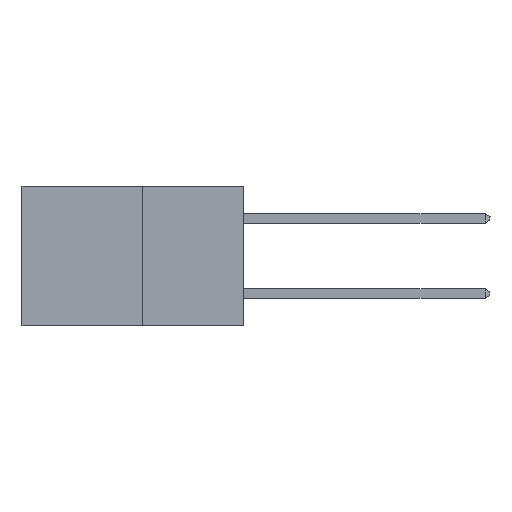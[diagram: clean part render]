
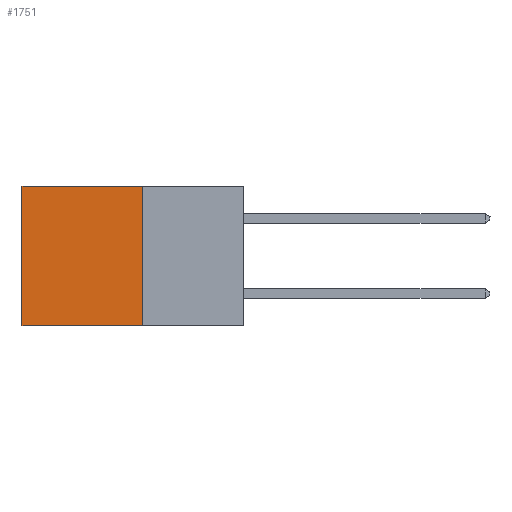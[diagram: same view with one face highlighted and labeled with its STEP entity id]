
A CAD part, left-side view. The second image highlights one B-rep face of the part: STEP entity #1751.
In plain terms, the highlighted planar face has unit normal (-1, 0, 0).
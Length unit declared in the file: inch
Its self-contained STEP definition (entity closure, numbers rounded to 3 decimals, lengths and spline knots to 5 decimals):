
#308 = CARTESIAN_POINT ( 'NONE',  ( 0.277, 0.59, -0.37 ) ) ;
#325 = EDGE_LOOP ( 'NONE', ( #4494, #8469, #2563, #4719 ) ) ;
#544 = DIRECTION ( 'NONE',  ( 0., 1., 0. ) ) ;
#680 = EDGE_CURVE ( 'NONE', #7428, #1618, #8091, .T. ) ;
#886 = CARTESIAN_POINT ( 'NONE',  ( 0.277, 0.27, 0. ) ) ;
#1152 = VECTOR ( 'NONE', #3304, 39.37008 ) ;
#1618 = VERTEX_POINT ( 'NONE', #3515 ) ;
#1751 = ADVANCED_FACE ( 'NONE', ( #7575 ), #4435, .F. ) ;
#1861 = VECTOR ( 'NONE', #5098, 39.37008 ) ;
#1868 = LINE ( 'NONE', #4894, #5915 ) ;
#2135 = CARTESIAN_POINT ( 'NONE',  ( 0.277, 0.27, -0.37 ) ) ;
#2257 = EDGE_CURVE ( 'NONE', #8709, #5207, #7914, .T. ) ;
#2388 = CARTESIAN_POINT ( 'NONE',  ( 0.277, 0.59, 0. ) ) ;
#2563 = ORIENTED_EDGE ( 'NONE', *, *, #680, .F. ) ;
#3304 = DIRECTION ( 'NONE',  ( 0., 0., -1. ) ) ;
#3515 = CARTESIAN_POINT ( 'NONE',  ( 0.277, 0.27, -0.37 ) ) ;
#4188 = DIRECTION ( 'NONE',  ( 0., 0., -1. ) ) ;
#4197 = DIRECTION ( 'NONE',  ( 1., 0., 0. ) ) ;
#4217 = CARTESIAN_POINT ( 'NONE',  ( 0.277, 0.27, -0.37 ) ) ;
#4435 = PLANE ( 'NONE',  #8001 ) ;
#4494 = ORIENTED_EDGE ( 'NONE', *, *, #2257, .T. ) ;
#4719 = ORIENTED_EDGE ( 'NONE', *, *, #7947, .T. ) ;
#4894 = CARTESIAN_POINT ( 'NONE',  ( 0.277, 0.27, -0.37 ) ) ;
#4993 = DIRECTION ( 'NONE',  ( 0., 1., 0. ) ) ;
#5098 = DIRECTION ( 'NONE',  ( 0., 0., -1. ) ) ;
#5207 = VERTEX_POINT ( 'NONE', #6485 ) ;
#5904 = VECTOR ( 'NONE', #544, 39.37008 ) ;
#5915 = VECTOR ( 'NONE', #4993, 39.37008 ) ;
#6138 = LINE ( 'NONE', #9178, #5904 ) ;
#6485 = CARTESIAN_POINT ( 'NONE',  ( 0.277, 0.59, -0.37 ) ) ;
#6603 = EDGE_CURVE ( 'NONE', #1618, #5207, #1868, .T. ) ;
#7428 = VERTEX_POINT ( 'NONE', #886 ) ;
#7575 = FACE_OUTER_BOUND ( 'NONE', #325, .T. ) ;
#7914 = LINE ( 'NONE', #308, #1152 ) ;
#7947 = EDGE_CURVE ( 'NONE', #7428, #8709, #6138, .T. ) ;
#8001 = AXIS2_PLACEMENT_3D ( 'NONE', #4217, #4197, #4188 ) ;
#8091 = LINE ( 'NONE', #2135, #1861 ) ;
#8469 = ORIENTED_EDGE ( 'NONE', *, *, #6603, .F. ) ;
#8709 = VERTEX_POINT ( 'NONE', #2388 ) ;
#9178 = CARTESIAN_POINT ( 'NONE',  ( 0.277, 0.27, 0. ) ) ;
